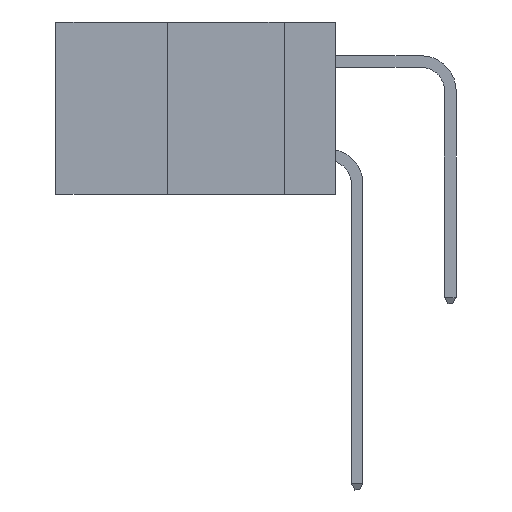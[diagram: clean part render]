
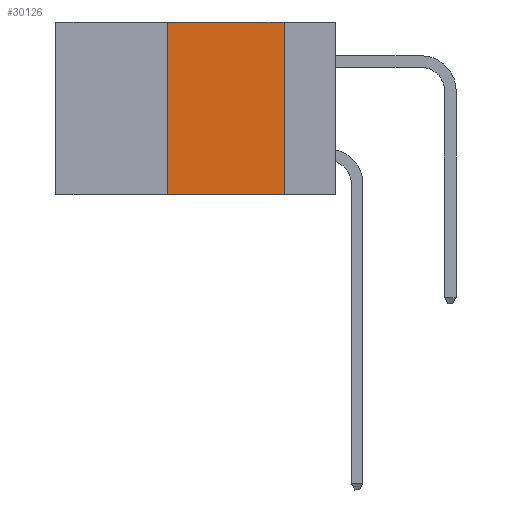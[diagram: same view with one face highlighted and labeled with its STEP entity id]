
A CAD part, left-side view. The second image highlights one B-rep face of the part: STEP entity #30126.
In plain terms, the highlighted planar face has unit normal (-1, 0, 0).
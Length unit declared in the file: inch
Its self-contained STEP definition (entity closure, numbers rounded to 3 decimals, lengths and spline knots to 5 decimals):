
#2677 = LINE ( 'NONE', #15298, #20196 ) ;
#2702 = FACE_OUTER_BOUND ( 'NONE', #10103, .T. ) ;
#2759 = EDGE_CURVE ( 'NONE', #23808, #11964, #17000, .T. ) ;
#3261 = VECTOR ( 'NONE', #8396, 39.37008 ) ;
#3761 = VERTEX_POINT ( 'NONE', #26512 ) ;
#3773 = ORIENTED_EDGE ( 'NONE', *, *, #2759, .F. ) ;
#4457 = LINE ( 'NONE', #31238, #12461 ) ;
#6497 = DIRECTION ( 'NONE',  ( 0., 0., -1. ) ) ;
#6943 = CARTESIAN_POINT ( 'NONE',  ( 0., 0.36, 0. ) ) ;
#7797 = CARTESIAN_POINT ( 'NONE',  ( 0., 0.36, -0.37 ) ) ;
#8396 = DIRECTION ( 'NONE',  ( 0., 0., 1. ) ) ;
#8706 = DIRECTION ( 'NONE',  ( 1., 0., 0. ) ) ;
#10103 = EDGE_LOOP ( 'NONE', ( #29104, #11688, #3773, #10456 ) ) ;
#10456 = ORIENTED_EDGE ( 'NONE', *, *, #15171, .T. ) ;
#11688 = ORIENTED_EDGE ( 'NONE', *, *, #26008, .F. ) ;
#11964 = VERTEX_POINT ( 'NONE', #6943 ) ;
#12461 = VECTOR ( 'NONE', #24768, 39.37008 ) ;
#12978 = CARTESIAN_POINT ( 'NONE',  ( 0., 0.11, -0.37 ) ) ;
#13278 = VECTOR ( 'NONE', #20384, 39.37008 ) ;
#13424 = CARTESIAN_POINT ( 'NONE',  ( 0., 0.36, 0. ) ) ;
#13709 = PLANE ( 'NONE',  #17676 ) ;
#15171 = EDGE_CURVE ( 'NONE', #23808, #28612, #4457, .T. ) ;
#15298 = CARTESIAN_POINT ( 'NONE',  ( 0., 0.11, 0. ) ) ;
#16468 = CARTESIAN_POINT ( 'NONE',  ( 0., 0.6, 0. ) ) ;
#17000 = LINE ( 'NONE', #13424, #3261 ) ;
#17676 = AXIS2_PLACEMENT_3D ( 'NONE', #16468, #8706, #6497 ) ;
#17732 = DIRECTION ( 'NONE',  ( 0., 0., -1. ) ) ;
#19477 = EDGE_CURVE ( 'NONE', #3761, #28612, #2677, .T. ) ;
#19744 = LINE ( 'NONE', #20729, #13278 ) ;
#20196 = VECTOR ( 'NONE', #17732, 39.37008 ) ;
#20384 = DIRECTION ( 'NONE',  ( 0., -1., 0. ) ) ;
#20729 = CARTESIAN_POINT ( 'NONE',  ( 0., 0.6, 0. ) ) ;
#23808 = VERTEX_POINT ( 'NONE', #7797 ) ;
#24768 = DIRECTION ( 'NONE',  ( 0., -1., 0. ) ) ;
#26008 = EDGE_CURVE ( 'NONE', #11964, #3761, #19744, .T. ) ;
#26512 = CARTESIAN_POINT ( 'NONE',  ( 0., 0.11, 0. ) ) ;
#28612 = VERTEX_POINT ( 'NONE', #12978 ) ;
#29104 = ORIENTED_EDGE ( 'NONE', *, *, #19477, .F. ) ;
#30126 = ADVANCED_FACE ( 'NONE', ( #2702 ), #13709, .F. ) ;
#31238 = CARTESIAN_POINT ( 'NONE',  ( 0., 0.6, -0.37 ) ) ;
